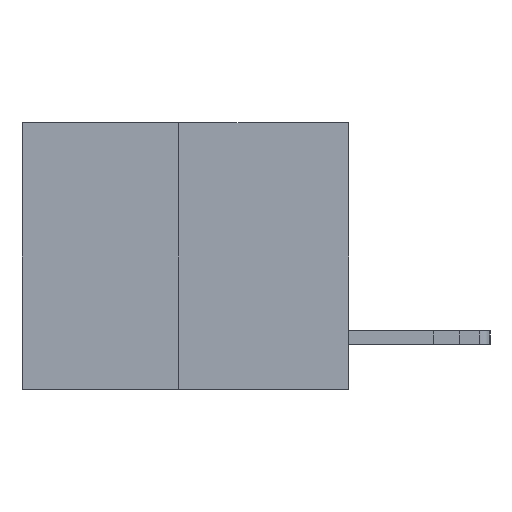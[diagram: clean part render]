
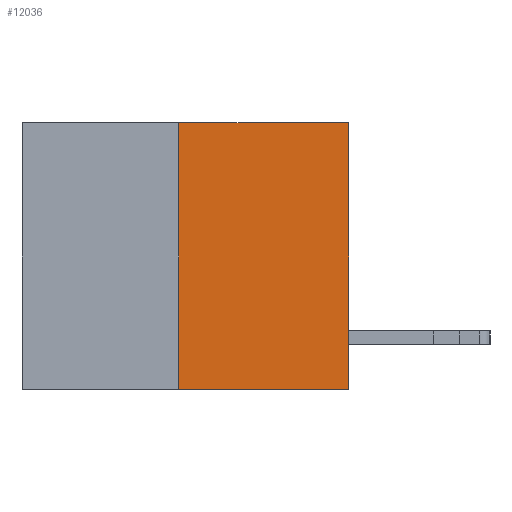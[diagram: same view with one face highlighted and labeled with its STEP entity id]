
A CAD part, left-side view. The second image highlights one B-rep face of the part: STEP entity #12036.
In plain terms, the highlighted planar face has unit normal (-1, 0, 0).
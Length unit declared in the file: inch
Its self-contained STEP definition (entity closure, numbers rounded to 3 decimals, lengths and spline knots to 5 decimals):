
#277 = PLANE ( 'NONE',  #13971 ) ;
#883 = EDGE_CURVE ( 'NONE', #1670, #1414, #15073, .T. ) ;
#1300 = ORIENTED_EDGE ( 'NONE', *, *, #883, .F. ) ;
#1414 = VERTEX_POINT ( 'NONE', #11747 ) ;
#1553 = LINE ( 'NONE', #9860, #9814 ) ;
#1592 = DIRECTION ( 'NONE',  ( 0., 0., 1. ) ) ;
#1624 = VECTOR ( 'NONE', #1802, 39.37008 ) ;
#1670 = VERTEX_POINT ( 'NONE', #9019 ) ;
#1711 = DIRECTION ( 'NONE',  ( 0., 0., -1. ) ) ;
#1802 = DIRECTION ( 'NONE',  ( 0., 0., 1. ) ) ;
#2588 = LINE ( 'NONE', #3974, #6303 ) ;
#2967 = CARTESIAN_POINT ( 'NONE',  ( 0., 0.6, 0. ) ) ;
#3974 = CARTESIAN_POINT ( 'NONE',  ( 0., 0.6, -0.49 ) ) ;
#4367 = DIRECTION ( 'NONE',  ( 0., -1., 0. ) ) ;
#4395 = VERTEX_POINT ( 'NONE', #9397 ) ;
#4730 = EDGE_CURVE ( 'NONE', #15300, #4395, #5096, .T. ) ;
#5096 = LINE ( 'NONE', #13721, #1624 ) ;
#5232 = DIRECTION ( 'NONE',  ( 0., -1., 0. ) ) ;
#6303 = VECTOR ( 'NONE', #5232, 39.37008 ) ;
#6452 = EDGE_CURVE ( 'NONE', #1414, #4395, #1553, .T. ) ;
#8293 = CARTESIAN_POINT ( 'NONE',  ( 0., 0.312, -0.49 ) ) ;
#9019 = CARTESIAN_POINT ( 'NONE',  ( 0., 0.312, -0.49 ) ) ;
#9186 = EDGE_LOOP ( 'NONE', ( #1300, #9242, #13923, #11904 ) ) ;
#9242 = ORIENTED_EDGE ( 'NONE', *, *, #14947, .T. ) ;
#9397 = CARTESIAN_POINT ( 'NONE',  ( 0., 0., 0. ) ) ;
#9814 = VECTOR ( 'NONE', #4367, 39.37008 ) ;
#9860 = CARTESIAN_POINT ( 'NONE',  ( 0., 0.6, 0. ) ) ;
#11510 = VECTOR ( 'NONE', #1592, 39.37008 ) ;
#11747 = CARTESIAN_POINT ( 'NONE',  ( 0., 0.312, 0. ) ) ;
#11904 = ORIENTED_EDGE ( 'NONE', *, *, #6452, .F. ) ;
#12036 = ADVANCED_FACE ( 'NONE', ( #15037 ), #277, .F. ) ;
#13721 = CARTESIAN_POINT ( 'NONE',  ( 0., 0., 0. ) ) ;
#13923 = ORIENTED_EDGE ( 'NONE', *, *, #4730, .T. ) ;
#13971 = AXIS2_PLACEMENT_3D ( 'NONE', #2967, #14836, #1711 ) ;
#14836 = DIRECTION ( 'NONE',  ( 1., 0., 0. ) ) ;
#14947 = EDGE_CURVE ( 'NONE', #1670, #15300, #2588, .T. ) ;
#15037 = FACE_OUTER_BOUND ( 'NONE', #9186, .T. ) ;
#15073 = LINE ( 'NONE', #8293, #11510 ) ;
#15300 = VERTEX_POINT ( 'NONE', #16302 ) ;
#16302 = CARTESIAN_POINT ( 'NONE',  ( 0., 0., -0.49 ) ) ;
